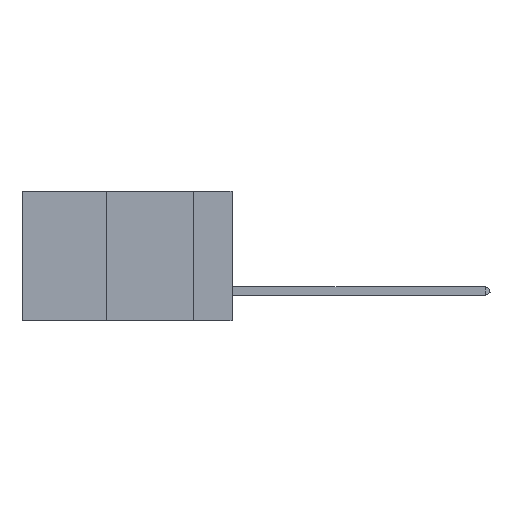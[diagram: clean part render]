
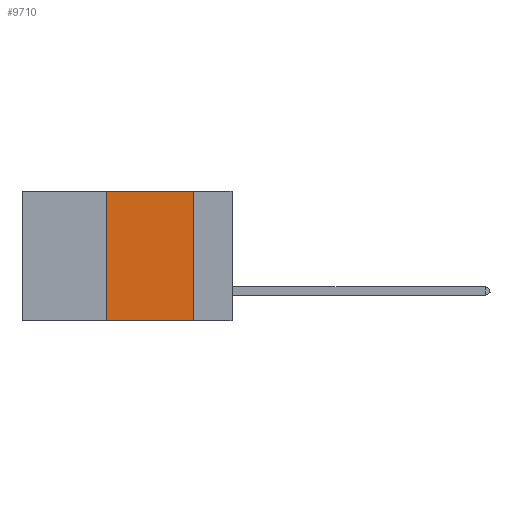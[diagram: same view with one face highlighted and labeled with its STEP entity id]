
A CAD part, left-side view. The second image highlights one B-rep face of the part: STEP entity #9710.
In plain terms, the highlighted planar face has unit normal (-1, 0, 0).
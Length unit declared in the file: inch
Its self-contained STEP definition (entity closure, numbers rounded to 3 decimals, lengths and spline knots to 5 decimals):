
#41 = DIRECTION ( 'NONE',  ( 0., -1., 0. ) ) ;
#542 = EDGE_CURVE ( 'NONE', #5374, #18224, #19771, .T. ) ;
#933 = AXIS2_PLACEMENT_3D ( 'NONE', #5445, #13753, #20203 ) ;
#1967 = CARTESIAN_POINT ( 'NONE',  ( 0., 0.36, 0. ) ) ;
#2096 = VECTOR ( 'NONE', #19540, 39.37008 ) ;
#2514 = ORIENTED_EDGE ( 'NONE', *, *, #3635, .F. ) ;
#2931 = FACE_OUTER_BOUND ( 'NONE', #17874, .T. ) ;
#3030 = CARTESIAN_POINT ( 'NONE',  ( 0., 0.6, -0.37 ) ) ;
#3635 = EDGE_CURVE ( 'NONE', #18224, #15806, #20410, .T. ) ;
#3708 = LINE ( 'NONE', #17637, #2096 ) ;
#4549 = CARTESIAN_POINT ( 'NONE',  ( 0., 0.11, -0.37 ) ) ;
#5374 = VERTEX_POINT ( 'NONE', #19593 ) ;
#5445 = CARTESIAN_POINT ( 'NONE',  ( 0., 0.6, 0. ) ) ;
#7684 = VECTOR ( 'NONE', #41, 39.37008 ) ;
#7800 = VERTEX_POINT ( 'NONE', #4549 ) ;
#8806 = CARTESIAN_POINT ( 'NONE',  ( 0., 0.36, 0. ) ) ;
#8945 = DIRECTION ( 'NONE',  ( 0., 0., 1. ) ) ;
#9097 = VECTOR ( 'NONE', #8945, 39.37008 ) ;
#9710 = ADVANCED_FACE ( 'NONE', ( #2931 ), #11934, .F. ) ;
#10276 = EDGE_CURVE ( 'NONE', #15806, #7800, #3708, .T. ) ;
#11661 = ORIENTED_EDGE ( 'NONE', *, *, #542, .F. ) ;
#11934 = PLANE ( 'NONE',  #933 ) ;
#13753 = DIRECTION ( 'NONE',  ( 1., 0., 0. ) ) ;
#13768 = CARTESIAN_POINT ( 'NONE',  ( 0., 0.11, 0. ) ) ;
#14615 = DIRECTION ( 'NONE',  ( 0., -1., 0. ) ) ;
#15806 = VERTEX_POINT ( 'NONE', #13768 ) ;
#16266 = LINE ( 'NONE', #3030, #18349 ) ;
#16594 = CARTESIAN_POINT ( 'NONE',  ( 0., 0.6, 0. ) ) ;
#17637 = CARTESIAN_POINT ( 'NONE',  ( 0., 0.11, 0. ) ) ;
#17874 = EDGE_LOOP ( 'NONE', ( #20568, #2514, #11661, #20528 ) ) ;
#18224 = VERTEX_POINT ( 'NONE', #1967 ) ;
#18349 = VECTOR ( 'NONE', #14615, 39.37008 ) ;
#19540 = DIRECTION ( 'NONE',  ( 0., 0., -1. ) ) ;
#19593 = CARTESIAN_POINT ( 'NONE',  ( 0., 0.36, -0.37 ) ) ;
#19599 = EDGE_CURVE ( 'NONE', #5374, #7800, #16266, .T. ) ;
#19771 = LINE ( 'NONE', #8806, #9097 ) ;
#20203 = DIRECTION ( 'NONE',  ( 0., 0., -1. ) ) ;
#20410 = LINE ( 'NONE', #16594, #7684 ) ;
#20528 = ORIENTED_EDGE ( 'NONE', *, *, #19599, .T. ) ;
#20568 = ORIENTED_EDGE ( 'NONE', *, *, #10276, .F. ) ;
